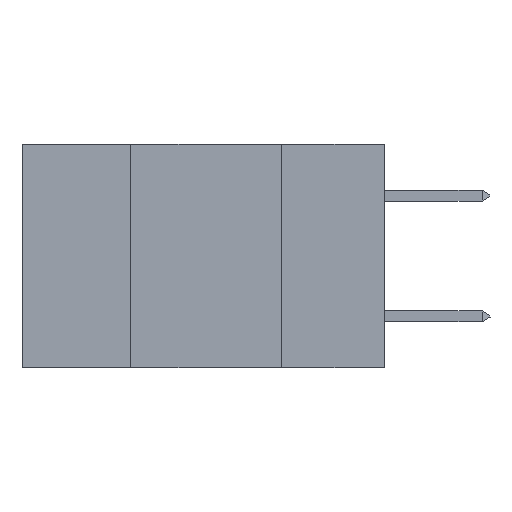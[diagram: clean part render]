
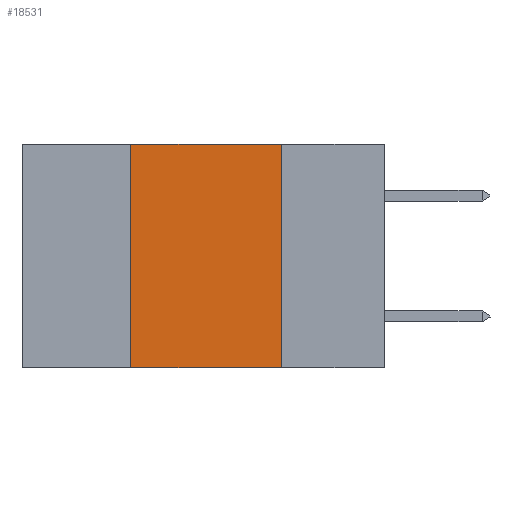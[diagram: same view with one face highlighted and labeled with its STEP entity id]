
A CAD part, left-side view. The second image highlights one B-rep face of the part: STEP entity #18531.
In plain terms, the highlighted planar face has unit normal (-1, 0, 0).
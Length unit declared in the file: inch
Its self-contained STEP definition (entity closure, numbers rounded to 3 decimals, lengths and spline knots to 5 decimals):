
#722 = EDGE_CURVE ( 'NONE', #9625, #17323, #6493, .T. ) ;
#886 = VECTOR ( 'NONE', #12045, 39.37008 ) ;
#1018 = DIRECTION ( 'NONE',  ( 0., 0., 1. ) ) ;
#1431 = ORIENTED_EDGE ( 'NONE', *, *, #1580, .F. ) ;
#1440 = CARTESIAN_POINT ( 'NONE',  ( 0., 0.6, -0.37 ) ) ;
#1580 = EDGE_CURVE ( 'NONE', #9625, #9045, #17105, .T. ) ;
#2051 = ORIENTED_EDGE ( 'NONE', *, *, #722, .T. ) ;
#2442 = VERTEX_POINT ( 'NONE', #3608 ) ;
#2809 = DIRECTION ( 'NONE',  ( 0., 0., -1. ) ) ;
#3479 = LINE ( 'NONE', #5768, #886 ) ;
#3608 = CARTESIAN_POINT ( 'NONE',  ( 0., 0.17, 0. ) ) ;
#3919 = CARTESIAN_POINT ( 'NONE',  ( 0., 0.6, 0. ) ) ;
#4339 = PLANE ( 'NONE',  #11018 ) ;
#4399 = VECTOR ( 'NONE', #13361, 39.37008 ) ;
#5151 = CARTESIAN_POINT ( 'NONE',  ( 0., 0.17, -0.37 ) ) ;
#5768 = CARTESIAN_POINT ( 'NONE',  ( 0., 0.17, 0. ) ) ;
#6235 = VECTOR ( 'NONE', #7395, 39.37008 ) ;
#6493 = LINE ( 'NONE', #1440, #4399 ) ;
#7006 = CARTESIAN_POINT ( 'NONE',  ( 0., 0.42, 0. ) ) ;
#7395 = DIRECTION ( 'NONE',  ( 0., -1., 0. ) ) ;
#7839 = LINE ( 'NONE', #15159, #6235 ) ;
#8142 = EDGE_CURVE ( 'NONE', #9045, #2442, #7839, .T. ) ;
#9045 = VERTEX_POINT ( 'NONE', #12822 ) ;
#9625 = VERTEX_POINT ( 'NONE', #13442 ) ;
#11018 = AXIS2_PLACEMENT_3D ( 'NONE', #3919, #17928, #2809 ) ;
#12045 = DIRECTION ( 'NONE',  ( 0., 0., -1. ) ) ;
#12822 = CARTESIAN_POINT ( 'NONE',  ( 0., 0.42, 0. ) ) ;
#13042 = EDGE_LOOP ( 'NONE', ( #18563, #13187, #1431, #2051 ) ) ;
#13187 = ORIENTED_EDGE ( 'NONE', *, *, #8142, .F. ) ;
#13361 = DIRECTION ( 'NONE',  ( 0., -1., 0. ) ) ;
#13442 = CARTESIAN_POINT ( 'NONE',  ( 0., 0.42, -0.37 ) ) ;
#14073 = FACE_OUTER_BOUND ( 'NONE', #13042, .T. ) ;
#15159 = CARTESIAN_POINT ( 'NONE',  ( 0., 0.6, 0. ) ) ;
#16152 = VECTOR ( 'NONE', #1018, 39.37008 ) ;
#17085 = EDGE_CURVE ( 'NONE', #2442, #17323, #3479, .T. ) ;
#17105 = LINE ( 'NONE', #7006, #16152 ) ;
#17323 = VERTEX_POINT ( 'NONE', #5151 ) ;
#17928 = DIRECTION ( 'NONE',  ( 1., 0., 0. ) ) ;
#18531 = ADVANCED_FACE ( 'NONE', ( #14073 ), #4339, .F. ) ;
#18563 = ORIENTED_EDGE ( 'NONE', *, *, #17085, .F. ) ;
